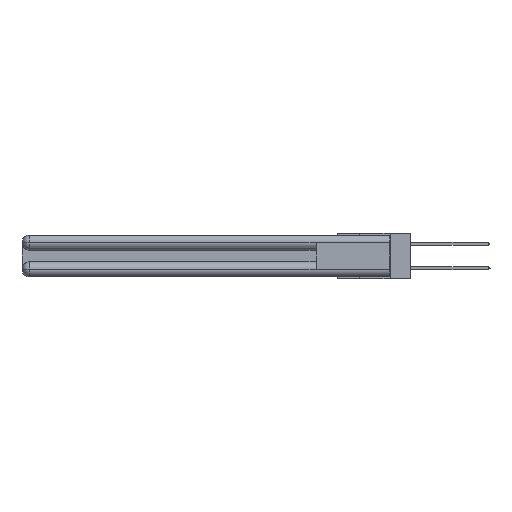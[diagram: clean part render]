
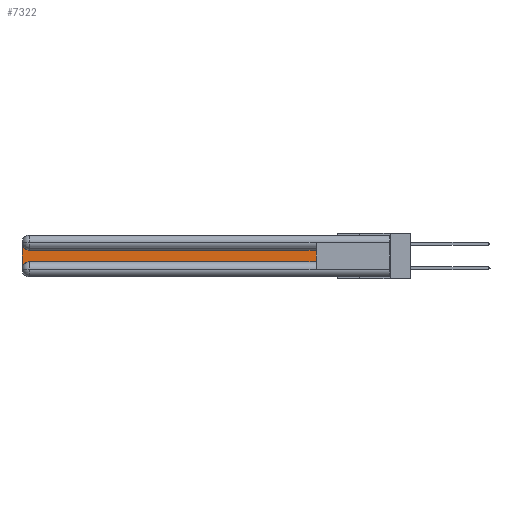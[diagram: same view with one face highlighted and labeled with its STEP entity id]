
A CAD part, left-side view. The second image highlights one B-rep face of the part: STEP entity #7322.
In plain terms, the highlighted planar face has unit normal (-1, 0, 0).
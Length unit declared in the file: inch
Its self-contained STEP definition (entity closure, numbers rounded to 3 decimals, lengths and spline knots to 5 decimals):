
#949 = CARTESIAN_POINT ( 'NONE',  ( 0.075, 0.6, -0.2175 ) ) ;
#1034 = CARTESIAN_POINT ( 'NONE',  ( 0.075, 3., -0.2775 ) ) ;
#1271 = EDGE_CURVE ( 'NONE', #12145, #14495, #30471, .T. ) ;
#1441 = DIRECTION ( 'NONE',  ( 0., 0., 1. ) ) ;
#3643 = DIRECTION ( 'NONE',  ( 1., 0., 0. ) ) ;
#5277 = CARTESIAN_POINT ( 'NONE',  ( 0.075, 0.6, -0.2175 ) ) ;
#5328 = VERTEX_POINT ( 'NONE', #21684 ) ;
#5338 = EDGE_CURVE ( 'NONE', #28243, #25091, #24796, .T. ) ;
#5460 = DIRECTION ( 'NONE',  ( 1., 0., 0. ) ) ;
#5723 = DIRECTION ( 'NONE',  ( 0., 0., -1. ) ) ;
#5911 = LINE ( 'NONE', #12258, #27499 ) ;
#6432 = VERTEX_POINT ( 'NONE', #14977 ) ;
#7322 = ADVANCED_FACE ( 'NONE', ( #22577 ), #22216, .F. ) ;
#7516 = ORIENTED_EDGE ( 'NONE', *, *, #27268, .T. ) ;
#8560 = CARTESIAN_POINT ( 'NONE',  ( 0.075, 2.94, -0.2175 ) ) ;
#8932 = DIRECTION ( 'NONE',  ( 0., 1., 0. ) ) ;
#9902 = AXIS2_PLACEMENT_3D ( 'NONE', #12956, #5460, #29608 ) ;
#11070 = VECTOR ( 'NONE', #1441, 39.37008 ) ;
#12145 = VERTEX_POINT ( 'NONE', #19163 ) ;
#12258 = CARTESIAN_POINT ( 'NONE',  ( 0.075, 3., -0.2175 ) ) ;
#12956 = CARTESIAN_POINT ( 'NONE',  ( 0.075, 3., -0.1225 ) ) ;
#13415 = VECTOR ( 'NONE', #15371, 39.37008 ) ;
#13745 = EDGE_CURVE ( 'NONE', #25091, #6432, #13814, .T. ) ;
#13814 = LINE ( 'NONE', #5277, #13415 ) ;
#14495 = VERTEX_POINT ( 'NONE', #24257 ) ;
#14977 = CARTESIAN_POINT ( 'NONE',  ( 0.075, 0.6, -0.2175 ) ) ;
#15371 = DIRECTION ( 'NONE',  ( 0., -1., 0. ) ) ;
#15390 = AXIS2_PLACEMENT_3D ( 'NONE', #17799, #24981, #22697 ) ;
#17799 = CARTESIAN_POINT ( 'NONE',  ( 0.075, 2.94, -0.0625 ) ) ;
#19163 = CARTESIAN_POINT ( 'NONE',  ( 0.075, 0.6, -0.1225 ) ) ;
#20377 = VECTOR ( 'NONE', #8932, 39.37008 ) ;
#20842 = ORIENTED_EDGE ( 'NONE', *, *, #5338, .T. ) ;
#21684 = CARTESIAN_POINT ( 'NONE',  ( 0.075, 3., -0.0625 ) ) ;
#22216 = PLANE ( 'NONE',  #9902 ) ;
#22485 = CARTESIAN_POINT ( 'NONE',  ( 0.075, 2.94, -0.2775 ) ) ;
#22577 = FACE_OUTER_BOUND ( 'NONE', #26049, .T. ) ;
#22697 = DIRECTION ( 'NONE',  ( 0., 0., -1. ) ) ;
#23016 = EDGE_CURVE ( 'NONE', #6432, #12145, #28583, .T. ) ;
#24257 = CARTESIAN_POINT ( 'NONE',  ( 0.075, 2.94, -0.1225 ) ) ;
#24540 = ORIENTED_EDGE ( 'NONE', *, *, #1271, .T. ) ;
#24796 = CIRCLE ( 'NONE', #26583, 0.06 ) ;
#24904 = CIRCLE ( 'NONE', #15390, 0.06 ) ;
#24981 = DIRECTION ( 'NONE',  ( 1., 0., 0. ) ) ;
#25091 = VERTEX_POINT ( 'NONE', #8560 ) ;
#25648 = CARTESIAN_POINT ( 'NONE',  ( 0.075, 0.6, -0.1225 ) ) ;
#26049 = EDGE_LOOP ( 'NONE', ( #24540, #26065, #7516, #20842, #26971, #28297 ) ) ;
#26065 = ORIENTED_EDGE ( 'NONE', *, *, #28258, .T. ) ;
#26171 = DIRECTION ( 'NONE',  ( 0., 0., -1. ) ) ;
#26583 = AXIS2_PLACEMENT_3D ( 'NONE', #22485, #3643, #5723 ) ;
#26971 = ORIENTED_EDGE ( 'NONE', *, *, #13745, .T. ) ;
#27268 = EDGE_CURVE ( 'NONE', #5328, #28243, #5911, .T. ) ;
#27499 = VECTOR ( 'NONE', #26171, 39.37008 ) ;
#28243 = VERTEX_POINT ( 'NONE', #1034 ) ;
#28258 = EDGE_CURVE ( 'NONE', #14495, #5328, #24904, .T. ) ;
#28297 = ORIENTED_EDGE ( 'NONE', *, *, #23016, .T. ) ;
#28583 = LINE ( 'NONE', #949, #11070 ) ;
#29608 = DIRECTION ( 'NONE',  ( 0., 0., -1. ) ) ;
#30471 = LINE ( 'NONE', #25648, #20377 ) ;
